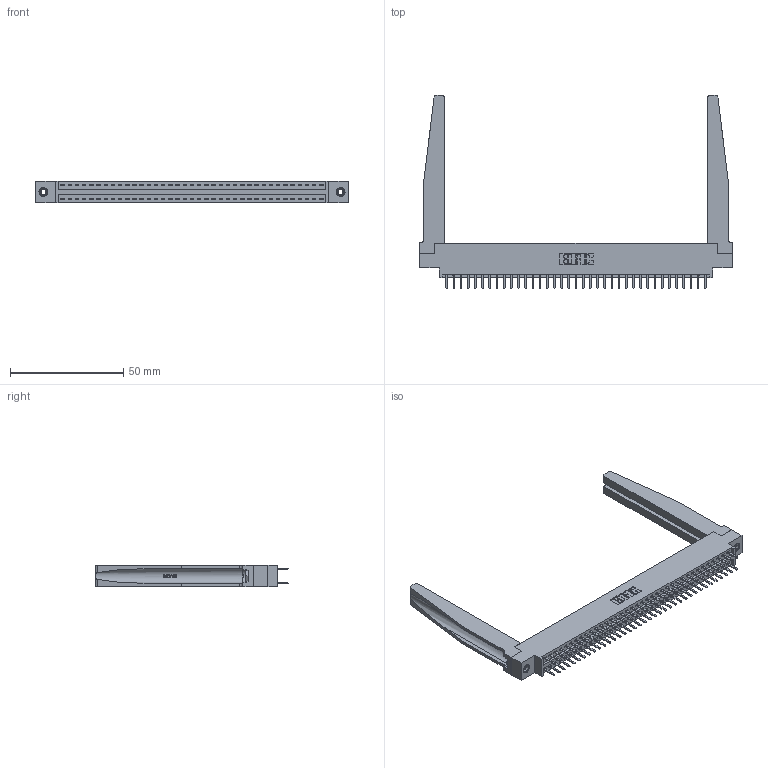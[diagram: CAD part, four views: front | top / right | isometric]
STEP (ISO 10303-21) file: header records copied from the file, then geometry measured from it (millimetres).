
FILE_DESCRIPTION (( 'STEP AP203' ), '1' );
FILE_NAME ('396-074-520-878.STEP', '2019-11-02T12:31:13', ( '' ), ( '' ), 'SwSTEP 2.0', 'SolidWorks 2016', '' );
FILE_SCHEMA (( 'CONFIG_CONTROL_DESIGN' ));
Length unit declared in the file: inch
Products named in the file (5): 345-250-001_345-250-001-102; 396-074-520-878; 346 Part_0.170 Offset - 0.156 Dia-TH; 345-292-001_345-293-120; 346-220-078_345-220-078
Assembly tree (79 placements, depth 2):
  396-074-520-878
    346 Part_0.170 Offset - 0.156 Dia-TH
    345-292-001_345-293-120  x74
    346-220-078_345-220-078  x2
    345-250-001_345-250-001-102  x2
Bounding box: 138.05 x 85.29 x 9.4 mm (x, y, z)
Volume: 20144.4 mm3; surface area: 24755.4 mm2
Topology: 79 solids, 79 shells, 4504 faces, 13011 edges, 8466 vertices
Faces by surface type: plane 2960, cylinder 1492, bspline 36, cone 12, torus 4
Entity records: 29814 total; most frequent: CARTESIAN_POINT 5871, ORIENTED_EDGE 4682, DIRECTION 4199, EDGE_CURVE 2341, LINE 1963, VECTOR 1963, VERTEX_POINT 1552, AXIS2_PLACEMENT_3D 1118
